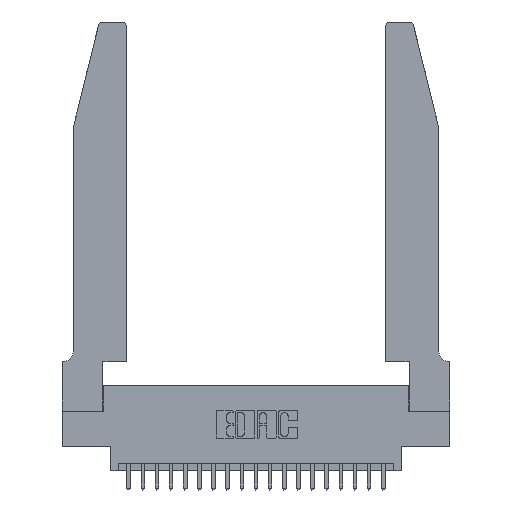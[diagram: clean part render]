
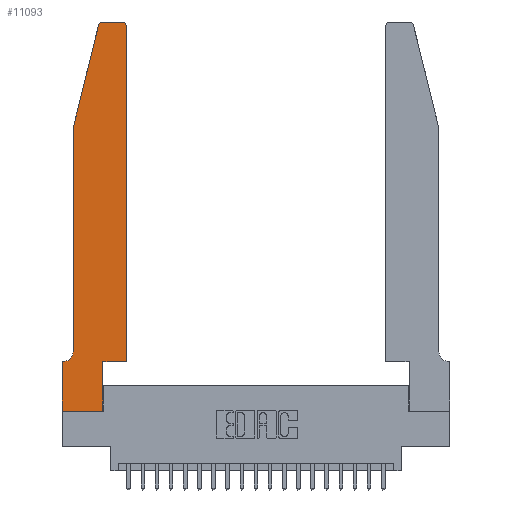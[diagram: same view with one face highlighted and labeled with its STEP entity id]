
A CAD part, top view. The second image highlights one B-rep face of the part: STEP entity #11093.
In plain terms, the highlighted planar face has unit normal (0, 0, 1).
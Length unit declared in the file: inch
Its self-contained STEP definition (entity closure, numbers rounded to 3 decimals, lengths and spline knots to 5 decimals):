
#51 = VERTEX_POINT ( 'NONE', #10343 ) ;
#104 = EDGE_CURVE ( 'NONE', #5190, #106, #18141, .T. ) ;
#106 = VERTEX_POINT ( 'NONE', #22724 ) ;
#184 = CIRCLE ( 'NONE', #1354, 0.03 ) ;
#254 = CARTESIAN_POINT ( 'NONE',  ( 0.0755, 0.42, 0.37 ) ) ;
#373 = VECTOR ( 'NONE', #4770, 39.37008 ) ;
#420 = CARTESIAN_POINT ( 'NONE',  ( 0., 0., 0.37 ) ) ;
#569 = CARTESIAN_POINT ( 'NONE',  ( 0.4505, 0.35, 0.37 ) ) ;
#881 = CARTESIAN_POINT ( 'NONE',  ( 0.0055, 0.35, 0.37 ) ) ;
#1060 = CARTESIAN_POINT ( 'NONE',  ( 0.0755, 2., 0.37 ) ) ;
#1109 = CARTESIAN_POINT ( 'NONE',  ( 0., 0., 0.37 ) ) ;
#1274 = VECTOR ( 'NONE', #3453, 39.37008 ) ;
#1354 = AXIS2_PLACEMENT_3D ( 'NONE', #4087, #16454, #5854 ) ;
#1650 = ORIENTED_EDGE ( 'NONE', *, *, #3774, .T. ) ;
#1687 = ORIENTED_EDGE ( 'NONE', *, *, #21594, .T. ) ;
#1697 = VERTEX_POINT ( 'NONE', #254 ) ;
#2357 = ORIENTED_EDGE ( 'NONE', *, *, #19830, .T. ) ;
#2480 = DIRECTION ( 'NONE',  ( -1., 0., 0. ) ) ;
#2533 = VECTOR ( 'NONE', #17052, 39.37008 ) ;
#2725 = EDGE_CURVE ( 'NONE', #16991, #51, #20075, .T. ) ;
#2914 = CARTESIAN_POINT ( 'NONE',  ( 0.0755, 2., 0.37 ) ) ;
#3453 = DIRECTION ( 'NONE',  ( 0., 1., 0. ) ) ;
#3774 = EDGE_CURVE ( 'NONE', #5606, #20071, #18416, .T. ) ;
#3775 = LINE ( 'NONE', #13168, #13230 ) ;
#4087 = CARTESIAN_POINT ( 'NONE',  ( 0.284, 2.72, 0.37 ) ) ;
#4608 = DIRECTION ( 'NONE',  ( 0., 0., -1. ) ) ;
#4623 = EDGE_CURVE ( 'NONE', #15392, #12626, #14618, .T. ) ;
#4770 = DIRECTION ( 'NONE',  ( 0., 1., 0. ) ) ;
#5040 = CARTESIAN_POINT ( 'NONE',  ( 0.4205, 2.75, 0.37 ) ) ;
#5041 = ORIENTED_EDGE ( 'NONE', *, *, #9298, .T. ) ;
#5190 = VERTEX_POINT ( 'NONE', #20468 ) ;
#5277 = DIRECTION ( 'NONE',  ( -1., 0., 0. ) ) ;
#5606 = VERTEX_POINT ( 'NONE', #14921 ) ;
#5689 = VERTEX_POINT ( 'NONE', #881 ) ;
#5854 = DIRECTION ( 'NONE',  ( 1., 0., 0. ) ) ;
#5996 = CARTESIAN_POINT ( 'NONE',  ( 0., 0.35, 0.37 ) ) ;
#6074 = DIRECTION ( 'NONE',  ( 1., 0., 0. ) ) ;
#6681 = DIRECTION ( 'NONE',  ( 0., 0., 1. ) ) ;
#6757 = CARTESIAN_POINT ( 'NONE',  ( 0.2865, 0., 0.37 ) ) ;
#7457 = EDGE_LOOP ( 'NONE', ( #19440, #17344, #11639, #13258, #5041, #1687, #1650, #2357, #9651, #22706, #11426, #21762 ) ) ;
#7650 = VECTOR ( 'NONE', #8209, 39.37008 ) ;
#7702 = CARTESIAN_POINT ( 'NONE',  ( 0.2865, 0.35, 0.37 ) ) ;
#7748 = VERTEX_POINT ( 'NONE', #5040 ) ;
#7938 = CARTESIAN_POINT ( 'NONE',  ( 0.4505, 0.35, 0.37 ) ) ;
#8209 = DIRECTION ( 'NONE',  ( 1., 0., 0. ) ) ;
#9123 = EDGE_CURVE ( 'NONE', #20469, #5190, #184, .T. ) ;
#9298 = EDGE_CURVE ( 'NONE', #1697, #5689, #11675, .T. ) ;
#9500 = CARTESIAN_POINT ( 'NONE',  ( 0.284, 2.75, 0.37 ) ) ;
#9651 = ORIENTED_EDGE ( 'NONE', *, *, #4623, .T. ) ;
#10343 = CARTESIAN_POINT ( 'NONE',  ( 0.4505, 2.72, 0.37 ) ) ;
#10656 = VECTOR ( 'NONE', #19334, 39.37008 ) ;
#11088 = EDGE_CURVE ( 'NONE', #7748, #20469, #3775, .T. ) ;
#11093 = ADVANCED_FACE ( 'NONE', ( #17339 ), #14948, .T. ) ;
#11426 = ORIENTED_EDGE ( 'NONE', *, *, #2725, .T. ) ;
#11568 = DIRECTION ( 'NONE',  ( -0.239, -0.971, 0. ) ) ;
#11639 = ORIENTED_EDGE ( 'NONE', *, *, #104, .T. ) ;
#11675 = CIRCLE ( 'NONE', #15663, 0.07 ) ;
#11877 = CARTESIAN_POINT ( 'NONE',  ( 0.2865, 0.35, 0.37 ) ) ;
#12626 = VERTEX_POINT ( 'NONE', #7702 ) ;
#12960 = VECTOR ( 'NONE', #11568, 39.37008 ) ;
#13168 = CARTESIAN_POINT ( 'NONE',  ( 0.2605, 2.75, 0.37 ) ) ;
#13230 = VECTOR ( 'NONE', #2480, 39.37008 ) ;
#13258 = ORIENTED_EDGE ( 'NONE', *, *, #21352, .T. ) ;
#13787 = VECTOR ( 'NONE', #21607, 39.37008 ) ;
#14369 = EDGE_CURVE ( 'NONE', #12626, #16991, #19941, .T. ) ;
#14618 = LINE ( 'NONE', #11877, #373 ) ;
#14921 = CARTESIAN_POINT ( 'NONE',  ( 0., 0.35, 0.37 ) ) ;
#14948 = PLANE ( 'NONE',  #19303 ) ;
#15234 = CARTESIAN_POINT ( 'NONE',  ( 0.0055, 0.42, 0.37 ) ) ;
#15358 = EDGE_CURVE ( 'NONE', #51, #7748, #18289, .T. ) ;
#15392 = VERTEX_POINT ( 'NONE', #6757 ) ;
#15663 = AXIS2_PLACEMENT_3D ( 'NONE', #15234, #4608, #16987 ) ;
#15905 = CARTESIAN_POINT ( 'NONE',  ( 0.0755, 0.35, 0.37 ) ) ;
#16407 = LINE ( 'NONE', #15905, #20488 ) ;
#16454 = DIRECTION ( 'NONE',  ( 0., 0., 1. ) ) ;
#16676 = DIRECTION ( 'NONE',  ( 0., 0., 1. ) ) ;
#16731 = CARTESIAN_POINT ( 'NONE',  ( 0.4505, 0.35, 0.37 ) ) ;
#16987 = DIRECTION ( 'NONE',  ( -1., 0., 0. ) ) ;
#16991 = VERTEX_POINT ( 'NONE', #7938 ) ;
#17052 = DIRECTION ( 'NONE',  ( 0., -1., 0. ) ) ;
#17240 = LINE ( 'NONE', #1060, #2533 ) ;
#17257 = CARTESIAN_POINT ( 'NONE',  ( 0.4205, 2.72, 0.37 ) ) ;
#17339 = FACE_OUTER_BOUND ( 'NONE', #7457, .T. ) ;
#17344 = ORIENTED_EDGE ( 'NONE', *, *, #9123, .T. ) ;
#18141 = LINE ( 'NONE', #2914, #12960 ) ;
#18289 = CIRCLE ( 'NONE', #18648, 0.03 ) ;
#18416 = LINE ( 'NONE', #420, #13787 ) ;
#18648 = AXIS2_PLACEMENT_3D ( 'NONE', #17257, #6681, #18990 ) ;
#18990 = DIRECTION ( 'NONE',  ( 1., 0., 0. ) ) ;
#19303 = AXIS2_PLACEMENT_3D ( 'NONE', #5996, #16676, #6074 ) ;
#19334 = DIRECTION ( 'NONE',  ( 1., 0., 0. ) ) ;
#19440 = ORIENTED_EDGE ( 'NONE', *, *, #11088, .T. ) ;
#19830 = EDGE_CURVE ( 'NONE', #20071, #15392, #21661, .T. ) ;
#19941 = LINE ( 'NONE', #569, #10656 ) ;
#20071 = VERTEX_POINT ( 'NONE', #1109 ) ;
#20075 = LINE ( 'NONE', #16731, #1274 ) ;
#20468 = CARTESIAN_POINT ( 'NONE',  ( 0.25487, 2.72718, 0.37 ) ) ;
#20469 = VERTEX_POINT ( 'NONE', #9500 ) ;
#20488 = VECTOR ( 'NONE', #5277, 39.37008 ) ;
#21352 = EDGE_CURVE ( 'NONE', #106, #1697, #17240, .T. ) ;
#21594 = EDGE_CURVE ( 'NONE', #5689, #5606, #16407, .T. ) ;
#21607 = DIRECTION ( 'NONE',  ( 0., -1., 0. ) ) ;
#21661 = LINE ( 'NONE', #22247, #7650 ) ;
#21762 = ORIENTED_EDGE ( 'NONE', *, *, #15358, .T. ) ;
#22247 = CARTESIAN_POINT ( 'NONE',  ( 0., 0., 0.37 ) ) ;
#22706 = ORIENTED_EDGE ( 'NONE', *, *, #14369, .T. ) ;
#22724 = CARTESIAN_POINT ( 'NONE',  ( 0.0755, 2., 0.37 ) ) ;
